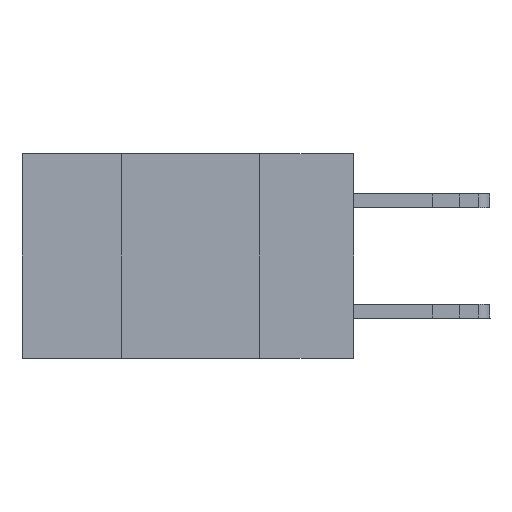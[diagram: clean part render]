
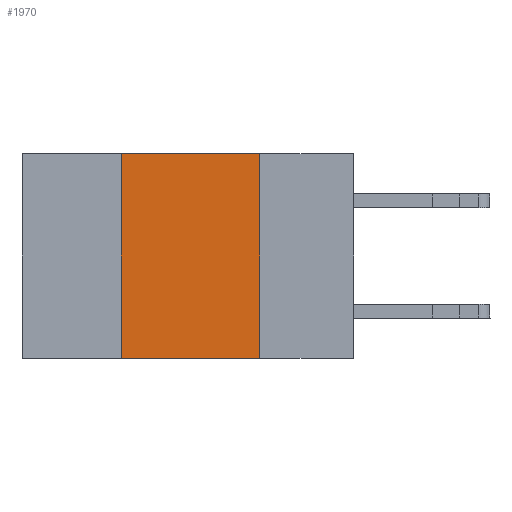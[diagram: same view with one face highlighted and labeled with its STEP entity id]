
A CAD part, left-side view. The second image highlights one B-rep face of the part: STEP entity #1970.
In plain terms, the highlighted planar face has unit normal (-1, 0, 0).
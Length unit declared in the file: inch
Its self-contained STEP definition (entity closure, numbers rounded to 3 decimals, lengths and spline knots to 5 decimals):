
#341 = LINE ( 'NONE', #1471, #7179 ) ;
#466 = LINE ( 'NONE', #11387, #14343 ) ;
#1319 = VECTOR ( 'NONE', #9996, 39.37008 ) ;
#1320 = PLANE ( 'NONE',  #4666 ) ;
#1471 = CARTESIAN_POINT ( 'NONE',  ( 0., 0.6, 0. ) ) ;
#1760 = LINE ( 'NONE', #13935, #1319 ) ;
#1970 = ADVANCED_FACE ( 'NONE', ( #3342 ), #1320, .F. ) ;
#2307 = CARTESIAN_POINT ( 'NONE',  ( 0., 0.17, 0. ) ) ;
#2696 = DIRECTION ( 'NONE',  ( 0., 0., -1. ) ) ;
#2791 = EDGE_CURVE ( 'NONE', #16125, #7068, #466, .T. ) ;
#3342 = FACE_OUTER_BOUND ( 'NONE', #15253, .T. ) ;
#3346 = CARTESIAN_POINT ( 'NONE',  ( 0., 0.42, -0.37 ) ) ;
#4666 = AXIS2_PLACEMENT_3D ( 'NONE', #15937, #10718, #2696 ) ;
#5254 = VERTEX_POINT ( 'NONE', #9860 ) ;
#6855 = EDGE_CURVE ( 'NONE', #9508, #5254, #14201, .T. ) ;
#6864 = DIRECTION ( 'NONE',  ( 0., -1., 0. ) ) ;
#7068 = VERTEX_POINT ( 'NONE', #9387 ) ;
#7155 = EDGE_CURVE ( 'NONE', #7068, #9508, #341, .T. ) ;
#7179 = VECTOR ( 'NONE', #6864, 39.37008 ) ;
#9387 = CARTESIAN_POINT ( 'NONE',  ( 0., 0.42, 0. ) ) ;
#9508 = VERTEX_POINT ( 'NONE', #2307 ) ;
#9860 = CARTESIAN_POINT ( 'NONE',  ( 0., 0.17, -0.37 ) ) ;
#9996 = DIRECTION ( 'NONE',  ( 0., -1., 0. ) ) ;
#10012 = DIRECTION ( 'NONE',  ( 0., 0., 1. ) ) ;
#10657 = VECTOR ( 'NONE', #15555, 39.37008 ) ;
#10718 = DIRECTION ( 'NONE',  ( 1., 0., 0. ) ) ;
#11387 = CARTESIAN_POINT ( 'NONE',  ( 0., 0.42, 0. ) ) ;
#12124 = ORIENTED_EDGE ( 'NONE', *, *, #6855, .F. ) ;
#12918 = ORIENTED_EDGE ( 'NONE', *, *, #7155, .F. ) ;
#12939 = ORIENTED_EDGE ( 'NONE', *, *, #2791, .F. ) ;
#13161 = ORIENTED_EDGE ( 'NONE', *, *, #16088, .T. ) ;
#13935 = CARTESIAN_POINT ( 'NONE',  ( 0., 0.6, -0.37 ) ) ;
#14201 = LINE ( 'NONE', #16805, #10657 ) ;
#14343 = VECTOR ( 'NONE', #10012, 39.37008 ) ;
#15253 = EDGE_LOOP ( 'NONE', ( #12124, #12918, #12939, #13161 ) ) ;
#15555 = DIRECTION ( 'NONE',  ( 0., 0., -1. ) ) ;
#15937 = CARTESIAN_POINT ( 'NONE',  ( 0., 0.6, 0. ) ) ;
#16088 = EDGE_CURVE ( 'NONE', #16125, #5254, #1760, .T. ) ;
#16125 = VERTEX_POINT ( 'NONE', #3346 ) ;
#16805 = CARTESIAN_POINT ( 'NONE',  ( 0., 0.17, 0. ) ) ;
